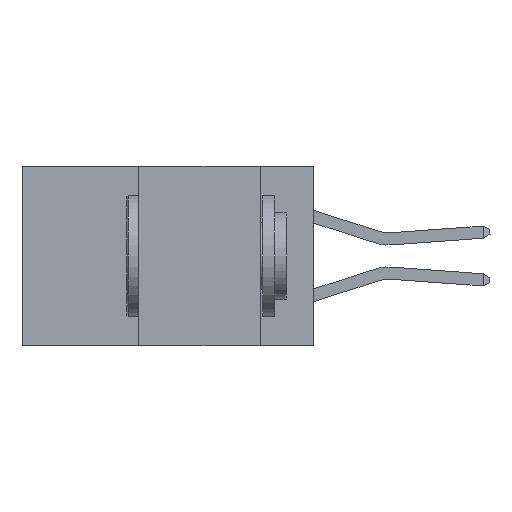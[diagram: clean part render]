
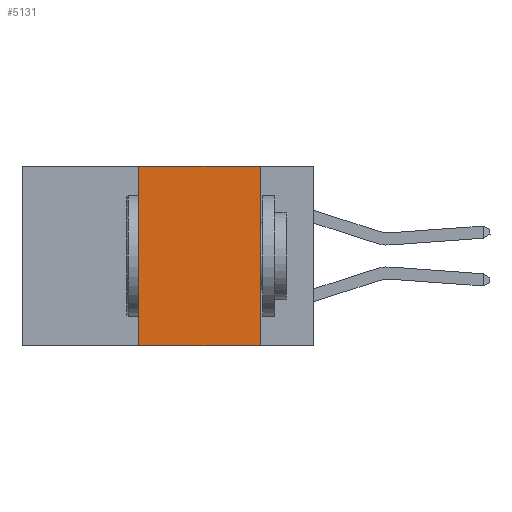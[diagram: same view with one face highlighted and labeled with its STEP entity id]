
A CAD part, left-side view. The second image highlights one B-rep face of the part: STEP entity #5131.
In plain terms, the highlighted planar face has unit normal (-1, 0, 0).
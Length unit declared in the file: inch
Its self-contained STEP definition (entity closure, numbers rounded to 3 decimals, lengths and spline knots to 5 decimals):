
#922 = DIRECTION ( 'NONE',  ( 0., -1., 0. ) ) ;
#3567 = DIRECTION ( 'NONE',  ( 1., 0., 0. ) ) ;
#4056 = LINE ( 'NONE', #10316, #20637 ) ;
#5131 = ADVANCED_FACE ( 'NONE', ( #7789 ), #36764, .F. ) ;
#6350 = VERTEX_POINT ( 'NONE', #39564 ) ;
#7789 = FACE_OUTER_BOUND ( 'NONE', #11082, .T. ) ;
#8580 = VERTEX_POINT ( 'NONE', #31808 ) ;
#9638 = LINE ( 'NONE', #38000, #42793 ) ;
#9764 = EDGE_CURVE ( 'NONE', #40651, #6350, #4056, .T. ) ;
#10316 = CARTESIAN_POINT ( 'NONE',  ( 0., 0.11, 0. ) ) ;
#11020 = LINE ( 'NONE', #21512, #12052 ) ;
#11082 = EDGE_LOOP ( 'NONE', ( #32492, #12810, #35083, #14362 ) ) ;
#12052 = VECTOR ( 'NONE', #24884, 39.37008 ) ;
#12810 = ORIENTED_EDGE ( 'NONE', *, *, #24597, .F. ) ;
#14362 = ORIENTED_EDGE ( 'NONE', *, *, #21891, .T. ) ;
#14978 = DIRECTION ( 'NONE',  ( 0., -1., 0. ) ) ;
#16117 = EDGE_CURVE ( 'NONE', #8580, #40694, #11020, .T. ) ;
#16153 = LINE ( 'NONE', #40683, #32706 ) ;
#16930 = DIRECTION ( 'NONE',  ( 0., 0., -1. ) ) ;
#16981 = DIRECTION ( 'NONE',  ( 0., 0., -1. ) ) ;
#20637 = VECTOR ( 'NONE', #16981, 39.37008 ) ;
#21377 = CARTESIAN_POINT ( 'NONE',  ( 0., 0.11, 0. ) ) ;
#21512 = CARTESIAN_POINT ( 'NONE',  ( 0., 0.36, 0. ) ) ;
#21521 = CARTESIAN_POINT ( 'NONE',  ( 0., 0.36, 0. ) ) ;
#21891 = EDGE_CURVE ( 'NONE', #8580, #6350, #9638, .T. ) ;
#24597 = EDGE_CURVE ( 'NONE', #40694, #40651, #16153, .T. ) ;
#24884 = DIRECTION ( 'NONE',  ( 0., 0., 1. ) ) ;
#31808 = CARTESIAN_POINT ( 'NONE',  ( 0., 0.36, -0.37 ) ) ;
#32492 = ORIENTED_EDGE ( 'NONE', *, *, #9764, .F. ) ;
#32706 = VECTOR ( 'NONE', #922, 39.37008 ) ;
#33421 = CARTESIAN_POINT ( 'NONE',  ( 0., 0.6, 0. ) ) ;
#35083 = ORIENTED_EDGE ( 'NONE', *, *, #16117, .F. ) ;
#36764 = PLANE ( 'NONE',  #41223 ) ;
#38000 = CARTESIAN_POINT ( 'NONE',  ( 0., 0.6, -0.37 ) ) ;
#39564 = CARTESIAN_POINT ( 'NONE',  ( 0., 0.11, -0.37 ) ) ;
#40651 = VERTEX_POINT ( 'NONE', #21377 ) ;
#40683 = CARTESIAN_POINT ( 'NONE',  ( 0., 0.6, 0. ) ) ;
#40694 = VERTEX_POINT ( 'NONE', #21521 ) ;
#41223 = AXIS2_PLACEMENT_3D ( 'NONE', #33421, #3567, #16930 ) ;
#42793 = VECTOR ( 'NONE', #14978, 39.37008 ) ;
